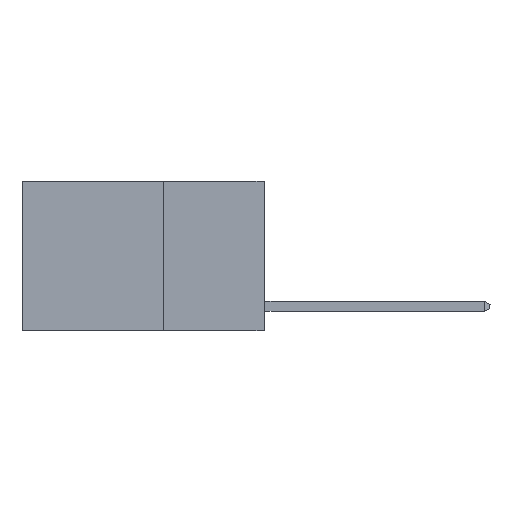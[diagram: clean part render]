
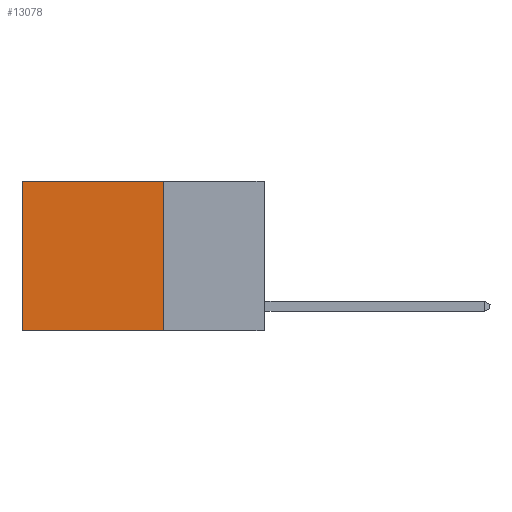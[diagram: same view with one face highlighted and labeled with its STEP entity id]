
A CAD part, left-side view. The second image highlights one B-rep face of the part: STEP entity #13078.
In plain terms, the highlighted planar face has unit normal (-1, 0, 0).
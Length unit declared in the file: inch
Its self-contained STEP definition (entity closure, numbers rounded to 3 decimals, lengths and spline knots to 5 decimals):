
#107 = ORIENTED_EDGE ( 'NONE', *, *, #13508, .T. ) ;
#283 = LINE ( 'NONE', #10621, #5826 ) ;
#1141 = VERTEX_POINT ( 'NONE', #12917 ) ;
#1881 = LINE ( 'NONE', #7033, #3028 ) ;
#1907 = EDGE_CURVE ( 'NONE', #15462, #8269, #283, .T. ) ;
#2544 = CARTESIAN_POINT ( 'NONE',  ( 0.2625, 0.25, 0. ) ) ;
#2798 = LINE ( 'NONE', #16694, #8470 ) ;
#3028 = VECTOR ( 'NONE', #12193, 39.37008 ) ;
#3289 = VECTOR ( 'NONE', #15631, 39.37008 ) ;
#4157 = DIRECTION ( 'NONE',  ( 0., 0., -1. ) ) ;
#5249 = LINE ( 'NONE', #9151, #3289 ) ;
#5826 = VECTOR ( 'NONE', #4157, 39.37008 ) ;
#6201 = DIRECTION ( 'NONE',  ( 0., 0., -1. ) ) ;
#6666 = CARTESIAN_POINT ( 'NONE',  ( 0.2625, 0.6, 0. ) ) ;
#7033 = CARTESIAN_POINT ( 'NONE',  ( 0.2625, 0.25, 0. ) ) ;
#8269 = VERTEX_POINT ( 'NONE', #12364 ) ;
#8470 = VECTOR ( 'NONE', #14098, 39.37008 ) ;
#9151 = CARTESIAN_POINT ( 'NONE',  ( 0.2625, 0.25, 0. ) ) ;
#9203 = ORIENTED_EDGE ( 'NONE', *, *, #13311, .F. ) ;
#10621 = CARTESIAN_POINT ( 'NONE',  ( 0.2625, 0.6, 0. ) ) ;
#10745 = CARTESIAN_POINT ( 'NONE',  ( 0.2625, 0.25, -0.37 ) ) ;
#11186 = EDGE_LOOP ( 'NONE', ( #11301, #16479, #9203, #107 ) ) ;
#11301 = ORIENTED_EDGE ( 'NONE', *, *, #1907, .T. ) ;
#11389 = VERTEX_POINT ( 'NONE', #10745 ) ;
#12193 = DIRECTION ( 'NONE',  ( 0., 1., 0. ) ) ;
#12364 = CARTESIAN_POINT ( 'NONE',  ( 0.2625, 0.6, -0.37 ) ) ;
#12917 = CARTESIAN_POINT ( 'NONE',  ( 0.2625, 0.25, 0. ) ) ;
#13078 = ADVANCED_FACE ( 'NONE', ( #16575 ), #14162, .F. ) ;
#13311 = EDGE_CURVE ( 'NONE', #1141, #11389, #5249, .T. ) ;
#13508 = EDGE_CURVE ( 'NONE', #1141, #15462, #1881, .T. ) ;
#14098 = DIRECTION ( 'NONE',  ( 0., 1., 0. ) ) ;
#14162 = PLANE ( 'NONE',  #16597 ) ;
#14251 = DIRECTION ( 'NONE',  ( 1., 0., 0. ) ) ;
#14441 = EDGE_CURVE ( 'NONE', #11389, #8269, #2798, .T. ) ;
#15462 = VERTEX_POINT ( 'NONE', #6666 ) ;
#15631 = DIRECTION ( 'NONE',  ( 0., 0., -1. ) ) ;
#16479 = ORIENTED_EDGE ( 'NONE', *, *, #14441, .F. ) ;
#16575 = FACE_OUTER_BOUND ( 'NONE', #11186, .T. ) ;
#16597 = AXIS2_PLACEMENT_3D ( 'NONE', #2544, #14251, #6201 ) ;
#16694 = CARTESIAN_POINT ( 'NONE',  ( 0.2625, 0.25, -0.37 ) ) ;
